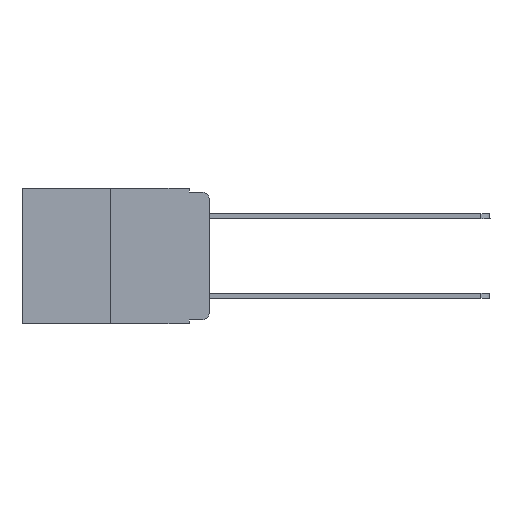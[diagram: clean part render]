
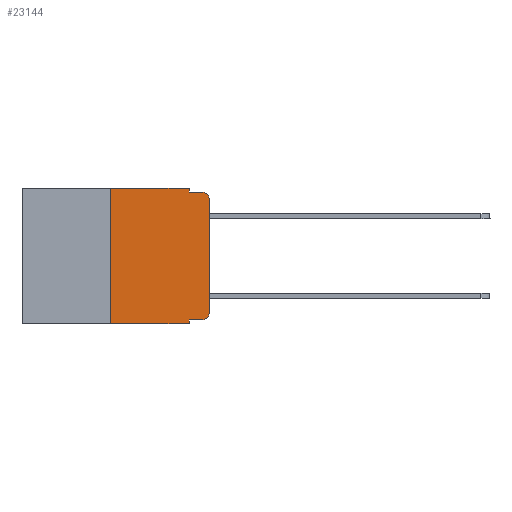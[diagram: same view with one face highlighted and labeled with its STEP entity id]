
A CAD part, left-side view. The second image highlights one B-rep face of the part: STEP entity #23144.
In plain terms, the highlighted planar face has unit normal (-1, 0, 0).
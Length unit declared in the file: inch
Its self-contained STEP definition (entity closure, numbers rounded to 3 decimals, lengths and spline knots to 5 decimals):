
#383 = DIRECTION ( 'NONE',  ( 0., -1., 0. ) ) ;
#590 = VECTOR ( 'NONE', #17890, 39.37008 ) ;
#812 = AXIS2_PLACEMENT_3D ( 'NONE', #6544, #4327, #22100 ) ;
#1398 = ORIENTED_EDGE ( 'NONE', *, *, #24751, .F. ) ;
#1485 = LINE ( 'NONE', #16545, #24256 ) ;
#1501 = AXIS2_PLACEMENT_3D ( 'NONE', #8480, #16453, #18324 ) ;
#2696 = DIRECTION ( 'NONE',  ( 0., 0., -1. ) ) ;
#2754 = VECTOR ( 'NONE', #10546, 39.37008 ) ;
#2932 = CARTESIAN_POINT ( 'NONE',  ( 0., 0.051, 0. ) ) ;
#3050 = VERTEX_POINT ( 'NONE', #14473 ) ;
#3158 = LINE ( 'NONE', #21633, #6199 ) ;
#3200 = ORIENTED_EDGE ( 'NONE', *, *, #4881, .T. ) ;
#3502 = EDGE_CURVE ( 'NONE', #7115, #13187, #17491, .T. ) ;
#3780 = VECTOR ( 'NONE', #12697, 39.37008 ) ;
#4161 = CARTESIAN_POINT ( 'NONE',  ( 0., 0.051, -0.333 ) ) ;
#4327 = DIRECTION ( 'NONE',  ( 1., 0., 0. ) ) ;
#4380 = LINE ( 'NONE', #8731, #3780 ) ;
#4413 = CARTESIAN_POINT ( 'NONE',  ( 0., 0.02, -0.333 ) ) ;
#4563 = VERTEX_POINT ( 'NONE', #5191 ) ;
#4573 = AXIS2_PLACEMENT_3D ( 'NONE', #23650, #7885, #5837 ) ;
#4881 = EDGE_CURVE ( 'NONE', #13770, #7115, #23220, .T. ) ;
#5051 = ORIENTED_EDGE ( 'NONE', *, *, #3502, .T. ) ;
#5124 = VERTEX_POINT ( 'NONE', #16435 ) ;
#5191 = CARTESIAN_POINT ( 'NONE',  ( 0., 0.25, -0.343 ) ) ;
#5382 = EDGE_CURVE ( 'NONE', #20976, #13383, #7920, .T. ) ;
#5837 = DIRECTION ( 'NONE',  ( 0., 0., -1. ) ) ;
#6199 = VECTOR ( 'NONE', #15621, 39.37008 ) ;
#6303 = VECTOR ( 'NONE', #10639, 39.37008 ) ;
#6534 = LINE ( 'NONE', #9543, #9886 ) ;
#6544 = CARTESIAN_POINT ( 'NONE',  ( 0., 0.473, 0. ) ) ;
#6622 = PLANE ( 'NONE',  #812 ) ;
#7115 = VERTEX_POINT ( 'NONE', #4413 ) ;
#7885 = DIRECTION ( 'NONE',  ( -1., 0., 0. ) ) ;
#7920 = LINE ( 'NONE', #18570, #2754 ) ;
#8140 = VECTOR ( 'NONE', #383, 39.37008 ) ;
#8480 = CARTESIAN_POINT ( 'NONE',  ( 0., 0.02, -0.03 ) ) ;
#8647 = CIRCLE ( 'NONE', #1501, 0.02 ) ;
#8731 = CARTESIAN_POINT ( 'NONE',  ( 0., 0.25, 0. ) ) ;
#8791 = ORIENTED_EDGE ( 'NONE', *, *, #22004, .F. ) ;
#9543 = CARTESIAN_POINT ( 'NONE',  ( 0., 0.473, -0.343 ) ) ;
#9606 = CARTESIAN_POINT ( 'NONE',  ( 0., 0.051, -0.333 ) ) ;
#9886 = VECTOR ( 'NONE', #23309, 39.37008 ) ;
#10546 = DIRECTION ( 'NONE',  ( 0., -1., 0. ) ) ;
#10639 = DIRECTION ( 'NONE',  ( 0., 0., -1. ) ) ;
#11008 = CARTESIAN_POINT ( 'NONE',  ( 0., 0., -0.313 ) ) ;
#11159 = EDGE_CURVE ( 'NONE', #13187, #5124, #25221, .T. ) ;
#11824 = EDGE_CURVE ( 'NONE', #15122, #20976, #1485, .T. ) ;
#12697 = DIRECTION ( 'NONE',  ( 0., 0., 1. ) ) ;
#12731 = VERTEX_POINT ( 'NONE', #17419 ) ;
#13187 = VERTEX_POINT ( 'NONE', #11008 ) ;
#13383 = VERTEX_POINT ( 'NONE', #16136 ) ;
#13770 = VERTEX_POINT ( 'NONE', #9606 ) ;
#14473 = CARTESIAN_POINT ( 'NONE',  ( 0., 0.25, 0. ) ) ;
#14782 = ORIENTED_EDGE ( 'NONE', *, *, #11824, .F. ) ;
#14952 = LINE ( 'NONE', #2932, #6303 ) ;
#15122 = VERTEX_POINT ( 'NONE', #24057 ) ;
#15621 = DIRECTION ( 'NONE',  ( 0., -1., 0. ) ) ;
#15729 = EDGE_CURVE ( 'NONE', #4563, #12731, #6534, .T. ) ;
#15878 = EDGE_CURVE ( 'NONE', #3050, #15122, #3158, .T. ) ;
#16136 = CARTESIAN_POINT ( 'NONE',  ( 0., 0.02, -0.01 ) ) ;
#16435 = CARTESIAN_POINT ( 'NONE',  ( 0., 0., -0.03 ) ) ;
#16453 = DIRECTION ( 'NONE',  ( -1., 0., 0. ) ) ;
#16491 = ORIENTED_EDGE ( 'NONE', *, *, #15878, .F. ) ;
#16523 = EDGE_CURVE ( 'NONE', #5124, #13383, #8647, .T. ) ;
#16545 = CARTESIAN_POINT ( 'NONE',  ( 0., 0.051, 0. ) ) ;
#16751 = FACE_OUTER_BOUND ( 'NONE', #25229, .T. ) ;
#17396 = ORIENTED_EDGE ( 'NONE', *, *, #15729, .T. ) ;
#17419 = CARTESIAN_POINT ( 'NONE',  ( 0., 0.051, -0.343 ) ) ;
#17491 = CIRCLE ( 'NONE', #4573, 0.02 ) ;
#17890 = DIRECTION ( 'NONE',  ( 0., 0., 1. ) ) ;
#18324 = DIRECTION ( 'NONE',  ( 0., 0., -1. ) ) ;
#18570 = CARTESIAN_POINT ( 'NONE',  ( 0., 0.051, -0.01 ) ) ;
#20976 = VERTEX_POINT ( 'NONE', #24995 ) ;
#21144 = CARTESIAN_POINT ( 'NONE',  ( 0., 0., 0. ) ) ;
#21633 = CARTESIAN_POINT ( 'NONE',  ( 0., 0.473, 0. ) ) ;
#22004 = EDGE_CURVE ( 'NONE', #13770, #12731, #14952, .T. ) ;
#22100 = DIRECTION ( 'NONE',  ( 0., 0., -1. ) ) ;
#23144 = ADVANCED_FACE ( 'NONE', ( #16751 ), #6622, .F. ) ;
#23220 = LINE ( 'NONE', #4161, #8140 ) ;
#23309 = DIRECTION ( 'NONE',  ( 0., -1., 0. ) ) ;
#23565 = ORIENTED_EDGE ( 'NONE', *, *, #16523, .T. ) ;
#23650 = CARTESIAN_POINT ( 'NONE',  ( 0., 0.02, -0.313 ) ) ;
#24057 = CARTESIAN_POINT ( 'NONE',  ( 0., 0.051, 0. ) ) ;
#24256 = VECTOR ( 'NONE', #2696, 39.37008 ) ;
#24694 = ORIENTED_EDGE ( 'NONE', *, *, #11159, .T. ) ;
#24751 = EDGE_CURVE ( 'NONE', #4563, #3050, #4380, .T. ) ;
#24995 = CARTESIAN_POINT ( 'NONE',  ( 0., 0.051, -0.01 ) ) ;
#25077 = ORIENTED_EDGE ( 'NONE', *, *, #5382, .F. ) ;
#25221 = LINE ( 'NONE', #21144, #590 ) ;
#25229 = EDGE_LOOP ( 'NONE', ( #24694, #23565, #25077, #14782, #16491, #1398, #17396, #8791, #3200, #5051 ) ) ;
